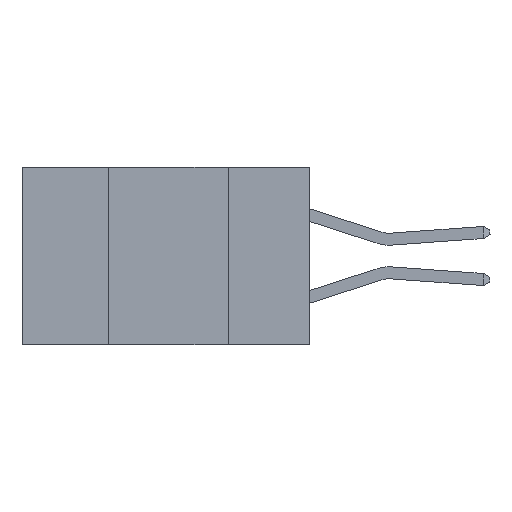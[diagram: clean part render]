
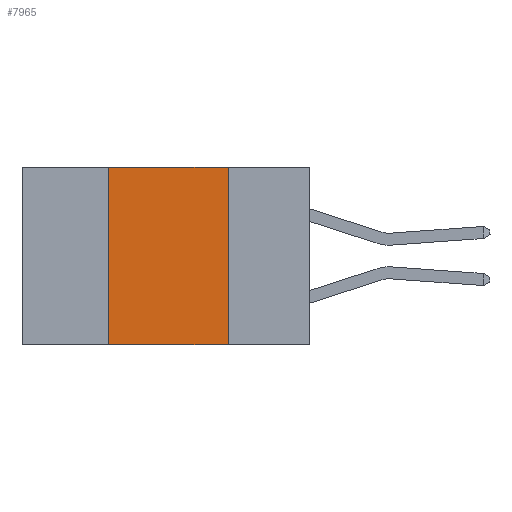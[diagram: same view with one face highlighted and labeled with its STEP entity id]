
A CAD part, left-side view. The second image highlights one B-rep face of the part: STEP entity #7965.
In plain terms, the highlighted planar face has unit normal (-1, 0, 0).
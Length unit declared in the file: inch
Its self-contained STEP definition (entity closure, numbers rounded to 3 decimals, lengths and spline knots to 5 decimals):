
#381 = PLANE ( 'NONE',  #27979 ) ;
#540 = DIRECTION ( 'NONE',  ( 0., -1., 0. ) ) ;
#2950 = CARTESIAN_POINT ( 'NONE',  ( 0., 0.6, -0.37 ) ) ;
#4034 = CARTESIAN_POINT ( 'NONE',  ( 0., 0.17, -0.37 ) ) ;
#4243 = EDGE_LOOP ( 'NONE', ( #19973, #27000, #8830, #21464 ) ) ;
#4726 = CARTESIAN_POINT ( 'NONE',  ( 0., 0.6, 0. ) ) ;
#4783 = CARTESIAN_POINT ( 'NONE',  ( 0., 0.17, 0. ) ) ;
#5207 = DIRECTION ( 'NONE',  ( 0., 0., -1. ) ) ;
#6197 = VERTEX_POINT ( 'NONE', #4034 ) ;
#6694 = VECTOR ( 'NONE', #21417, 39.37008 ) ;
#7965 = ADVANCED_FACE ( 'NONE', ( #10781 ), #381, .F. ) ;
#8727 = VERTEX_POINT ( 'NONE', #24404 ) ;
#8830 = ORIENTED_EDGE ( 'NONE', *, *, #28413, .F. ) ;
#9928 = CARTESIAN_POINT ( 'NONE',  ( 0., 0.6, 0. ) ) ;
#10313 = CARTESIAN_POINT ( 'NONE',  ( 0., 0.42, 0. ) ) ;
#10781 = FACE_OUTER_BOUND ( 'NONE', #4243, .T. ) ;
#12163 = CARTESIAN_POINT ( 'NONE',  ( 0., 0.17, 0. ) ) ;
#12313 = LINE ( 'NONE', #4783, #6694 ) ;
#12916 = VECTOR ( 'NONE', #26095, 39.37008 ) ;
#19048 = VERTEX_POINT ( 'NONE', #12163 ) ;
#19156 = EDGE_CURVE ( 'NONE', #8727, #6197, #28666, .T. ) ;
#19269 = DIRECTION ( 'NONE',  ( 0., 0., 1. ) ) ;
#19473 = DIRECTION ( 'NONE',  ( 1., 0., 0. ) ) ;
#19698 = EDGE_CURVE ( 'NONE', #23675, #19048, #26231, .T. ) ;
#19973 = ORIENTED_EDGE ( 'NONE', *, *, #23439, .F. ) ;
#21417 = DIRECTION ( 'NONE',  ( 0., 0., -1. ) ) ;
#21464 = ORIENTED_EDGE ( 'NONE', *, *, #19156, .T. ) ;
#22392 = VECTOR ( 'NONE', #540, 39.37008 ) ;
#23439 = EDGE_CURVE ( 'NONE', #19048, #6197, #12313, .T. ) ;
#23675 = VERTEX_POINT ( 'NONE', #10313 ) ;
#24404 = CARTESIAN_POINT ( 'NONE',  ( 0., 0.42, -0.37 ) ) ;
#24601 = VECTOR ( 'NONE', #19269, 39.37008 ) ;
#26095 = DIRECTION ( 'NONE',  ( 0., -1., 0. ) ) ;
#26231 = LINE ( 'NONE', #4726, #12916 ) ;
#27000 = ORIENTED_EDGE ( 'NONE', *, *, #19698, .F. ) ;
#27979 = AXIS2_PLACEMENT_3D ( 'NONE', #9928, #19473, #5207 ) ;
#28413 = EDGE_CURVE ( 'NONE', #8727, #23675, #30103, .T. ) ;
#28655 = CARTESIAN_POINT ( 'NONE',  ( 0., 0.42, 0. ) ) ;
#28666 = LINE ( 'NONE', #2950, #22392 ) ;
#30103 = LINE ( 'NONE', #28655, #24601 ) ;
